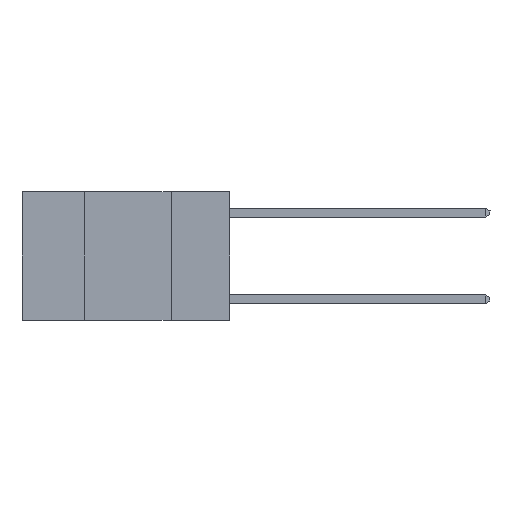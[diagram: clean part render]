
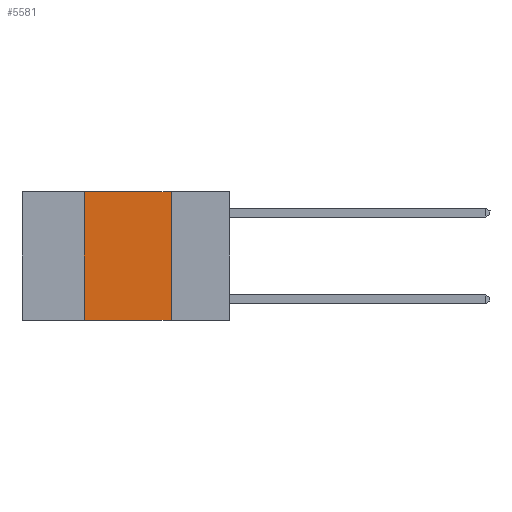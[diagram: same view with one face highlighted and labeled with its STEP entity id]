
A CAD part, left-side view. The second image highlights one B-rep face of the part: STEP entity #5581.
In plain terms, the highlighted planar face has unit normal (-1, 0, 0).
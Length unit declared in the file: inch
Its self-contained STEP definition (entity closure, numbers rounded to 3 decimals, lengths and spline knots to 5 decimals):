
#82 = CARTESIAN_POINT ( 'NONE',  ( 0., 0.6, 0. ) ) ;
#484 = EDGE_CURVE ( 'NONE', #6451, #5250, #5916, .T. ) ;
#1411 = ORIENTED_EDGE ( 'NONE', *, *, #8808, .T. ) ;
#1425 = CARTESIAN_POINT ( 'NONE',  ( 0., 0.17, -0.37 ) ) ;
#1485 = LINE ( 'NONE', #1724, #7470 ) ;
#1695 = PLANE ( 'NONE',  #4003 ) ;
#1724 = CARTESIAN_POINT ( 'NONE',  ( 0., 0.17, 0. ) ) ;
#1795 = VERTEX_POINT ( 'NONE', #6998 ) ;
#2138 = DIRECTION ( 'NONE',  ( 0., 0., 1. ) ) ;
#3032 = VERTEX_POINT ( 'NONE', #1425 ) ;
#3108 = DIRECTION ( 'NONE',  ( 0., -1., 0. ) ) ;
#3203 = CARTESIAN_POINT ( 'NONE',  ( 0., 0.6, 0. ) ) ;
#3236 = DIRECTION ( 'NONE',  ( 0., -1., 0. ) ) ;
#3334 = CARTESIAN_POINT ( 'NONE',  ( 0., 0.42, 0. ) ) ;
#3858 = CARTESIAN_POINT ( 'NONE',  ( 0., 0.42, 0. ) ) ;
#3864 = CARTESIAN_POINT ( 'NONE',  ( 0., 0.42, -0.37 ) ) ;
#4001 = DIRECTION ( 'NONE',  ( 0., 0., -1. ) ) ;
#4003 = AXIS2_PLACEMENT_3D ( 'NONE', #3203, #8687, #4001 ) ;
#4007 = VECTOR ( 'NONE', #3108, 39.37008 ) ;
#4040 = CARTESIAN_POINT ( 'NONE',  ( 0., 0.6, -0.37 ) ) ;
#4949 = ORIENTED_EDGE ( 'NONE', *, *, #5594, .F. ) ;
#5250 = VERTEX_POINT ( 'NONE', #3334 ) ;
#5546 = EDGE_CURVE ( 'NONE', #5250, #1795, #7137, .T. ) ;
#5581 = ADVANCED_FACE ( 'NONE', ( #9495 ), #1695, .F. ) ;
#5594 = EDGE_CURVE ( 'NONE', #1795, #3032, #1485, .T. ) ;
#5916 = LINE ( 'NONE', #3858, #7795 ) ;
#6451 = VERTEX_POINT ( 'NONE', #3864 ) ;
#6572 = ORIENTED_EDGE ( 'NONE', *, *, #5546, .F. ) ;
#6998 = CARTESIAN_POINT ( 'NONE',  ( 0., 0.17, 0. ) ) ;
#7137 = LINE ( 'NONE', #82, #4007 ) ;
#7190 = DIRECTION ( 'NONE',  ( 0., 0., -1. ) ) ;
#7470 = VECTOR ( 'NONE', #7190, 39.37008 ) ;
#7795 = VECTOR ( 'NONE', #2138, 39.37008 ) ;
#7888 = VECTOR ( 'NONE', #3236, 39.37008 ) ;
#8140 = ORIENTED_EDGE ( 'NONE', *, *, #484, .F. ) ;
#8687 = DIRECTION ( 'NONE',  ( 1., 0., 0. ) ) ;
#8808 = EDGE_CURVE ( 'NONE', #6451, #3032, #9653, .T. ) ;
#8825 = EDGE_LOOP ( 'NONE', ( #4949, #6572, #8140, #1411 ) ) ;
#9495 = FACE_OUTER_BOUND ( 'NONE', #8825, .T. ) ;
#9653 = LINE ( 'NONE', #4040, #7888 ) ;
